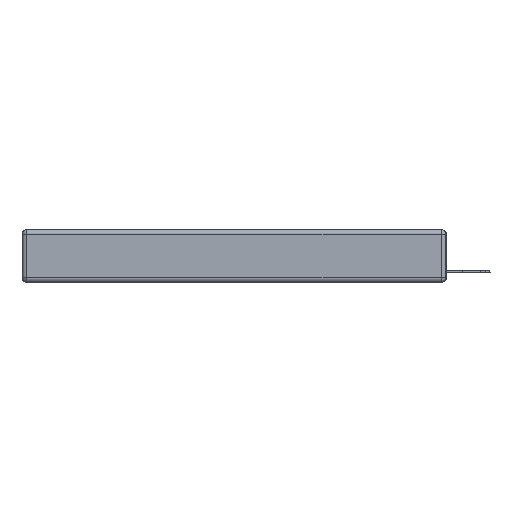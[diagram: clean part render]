
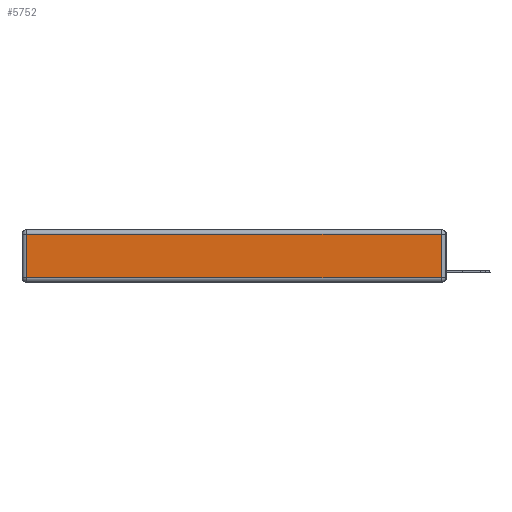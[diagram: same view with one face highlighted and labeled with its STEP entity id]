
A CAD part, left-side view. The second image highlights one B-rep face of the part: STEP entity #5752.
In plain terms, the highlighted planar face has unit normal (-1, 0, 0).
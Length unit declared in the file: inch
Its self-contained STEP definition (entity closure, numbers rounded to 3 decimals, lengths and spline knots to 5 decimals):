
#692 = VERTEX_POINT ( 'NONE', #1326 ) ;
#1326 = CARTESIAN_POINT ( 'NONE',  ( 0., 2.72, -0.313 ) ) ;
#1836 = EDGE_CURVE ( 'NONE', #8838, #26893, #20016, .T. ) ;
#1857 = CARTESIAN_POINT ( 'NONE',  ( 0., 2.75, -0.03 ) ) ;
#2239 = VECTOR ( 'NONE', #9924, 39.37008 ) ;
#3475 = VECTOR ( 'NONE', #8457, 39.37008 ) ;
#4293 = ORIENTED_EDGE ( 'NONE', *, *, #13455, .T. ) ;
#4616 = LINE ( 'NONE', #9825, #2239 ) ;
#4905 = CARTESIAN_POINT ( 'NONE',  ( 0., 0.03, -0.313 ) ) ;
#5752 = ADVANCED_FACE ( 'NONE', ( #22789 ), #20669, .T. ) ;
#7391 = AXIS2_PLACEMENT_3D ( 'NONE', #7575, #11878, #26878 ) ;
#7575 = CARTESIAN_POINT ( 'NONE',  ( 0., 0., -0.343 ) ) ;
#8457 = DIRECTION ( 'NONE',  ( 0., 1., 0. ) ) ;
#8838 = VERTEX_POINT ( 'NONE', #4905 ) ;
#9825 = CARTESIAN_POINT ( 'NONE',  ( 0., 2.72, -0.343 ) ) ;
#9924 = DIRECTION ( 'NONE',  ( 0., 0., -1. ) ) ;
#9926 = VERTEX_POINT ( 'NONE', #19622 ) ;
#11026 = CARTESIAN_POINT ( 'NONE',  ( 0., 0., -0.313 ) ) ;
#11878 = DIRECTION ( 'NONE',  ( -1., 0., 0. ) ) ;
#12668 = EDGE_CURVE ( 'NONE', #26893, #9926, #22514, .T. ) ;
#12734 = CARTESIAN_POINT ( 'NONE',  ( 0., 0.03, -0.343 ) ) ;
#12803 = VECTOR ( 'NONE', #16861, 39.37008 ) ;
#13455 = EDGE_CURVE ( 'NONE', #9926, #692, #4616, .T. ) ;
#14388 = ORIENTED_EDGE ( 'NONE', *, *, #19057, .T. ) ;
#15216 = EDGE_LOOP ( 'NONE', ( #14388, #17023, #15423, #4293 ) ) ;
#15423 = ORIENTED_EDGE ( 'NONE', *, *, #12668, .T. ) ;
#16861 = DIRECTION ( 'NONE',  ( 0., -1., 0. ) ) ;
#17023 = ORIENTED_EDGE ( 'NONE', *, *, #1836, .T. ) ;
#17150 = CARTESIAN_POINT ( 'NONE',  ( 0., 0.03, -0.03 ) ) ;
#18511 = LINE ( 'NONE', #11026, #12803 ) ;
#19057 = EDGE_CURVE ( 'NONE', #692, #8838, #18511, .T. ) ;
#19367 = DIRECTION ( 'NONE',  ( 0., 0., 1. ) ) ;
#19622 = CARTESIAN_POINT ( 'NONE',  ( 0., 2.72, -0.03 ) ) ;
#20016 = LINE ( 'NONE', #12734, #20682 ) ;
#20669 = PLANE ( 'NONE',  #7391 ) ;
#20682 = VECTOR ( 'NONE', #19367, 39.37008 ) ;
#22514 = LINE ( 'NONE', #1857, #3475 ) ;
#22789 = FACE_OUTER_BOUND ( 'NONE', #15216, .T. ) ;
#26878 = DIRECTION ( 'NONE',  ( 0., 0., 1. ) ) ;
#26893 = VERTEX_POINT ( 'NONE', #17150 ) ;
